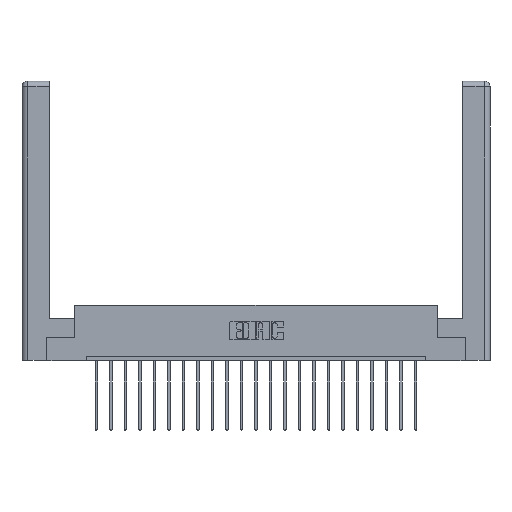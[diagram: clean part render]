
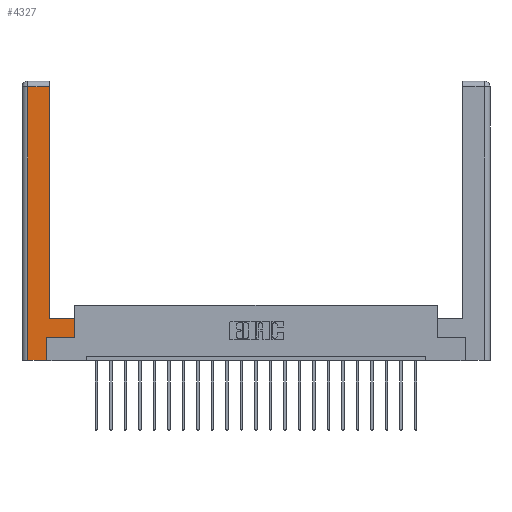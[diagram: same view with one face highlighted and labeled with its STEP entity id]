
A CAD part, top view. The second image highlights one B-rep face of the part: STEP entity #4327.
In plain terms, the highlighted planar face has unit normal (0, 0, 1).
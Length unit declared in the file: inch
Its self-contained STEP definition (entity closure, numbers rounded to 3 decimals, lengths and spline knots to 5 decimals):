
#248 = DIRECTION ( 'NONE',  ( -1., 0., 0. ) ) ;
#527 = DIRECTION ( 'NONE',  ( 1., 0., 0. ) ) ;
#644 = VERTEX_POINT ( 'NONE', #12038 ) ;
#904 = VERTEX_POINT ( 'NONE', #6009 ) ;
#1405 = ORIENTED_EDGE ( 'NONE', *, *, #10864, .T. ) ;
#1435 = CARTESIAN_POINT ( 'NONE',  ( 0.0615, 2.94, 0. ) ) ;
#1590 = LINE ( 'NONE', #9304, #5102 ) ;
#2837 = CARTESIAN_POINT ( 'NONE',  ( 0.295, 2.94, 0. ) ) ;
#3053 = VERTEX_POINT ( 'NONE', #1435 ) ;
#3635 = CARTESIAN_POINT ( 'NONE',  ( 0.0615, 2.94, 0. ) ) ;
#4297 = EDGE_CURVE ( 'NONE', #904, #19450, #11976, .T. ) ;
#4327 = ADVANCED_FACE ( 'NONE', ( #9293 ), #10858, .F. ) ;
#4337 = LINE ( 'NONE', #19168, #19892 ) ;
#4500 = ORIENTED_EDGE ( 'NONE', *, *, #20361, .T. ) ;
#5102 = VECTOR ( 'NONE', #7578, 39.37008 ) ;
#5104 = EDGE_CURVE ( 'NONE', #19450, #9506, #18352, .T. ) ;
#6009 = CARTESIAN_POINT ( 'NONE',  ( 0.265, 0., 0. ) ) ;
#6923 = CARTESIAN_POINT ( 'NONE',  ( 0.565, 0.45, 0. ) ) ;
#7255 = EDGE_LOOP ( 'NONE', ( #4500, #8034, #8121, #1405, #9281, #13465, #7885, #20680 ) ) ;
#7578 = DIRECTION ( 'NONE',  ( 0., 1., 0. ) ) ;
#7885 = ORIENTED_EDGE ( 'NONE', *, *, #19991, .T. ) ;
#8034 = ORIENTED_EDGE ( 'NONE', *, *, #12498, .T. ) ;
#8121 = ORIENTED_EDGE ( 'NONE', *, *, #20204, .T. ) ;
#8457 = CARTESIAN_POINT ( 'NONE',  ( 0.295, 0.45, 0. ) ) ;
#8510 = LINE ( 'NONE', #19008, #14132 ) ;
#8759 = VECTOR ( 'NONE', #17032, 39.37008 ) ;
#9281 = ORIENTED_EDGE ( 'NONE', *, *, #4297, .T. ) ;
#9293 = FACE_OUTER_BOUND ( 'NONE', #7255, .T. ) ;
#9304 = CARTESIAN_POINT ( 'NONE',  ( 0.295, 3., 0. ) ) ;
#9506 = VERTEX_POINT ( 'NONE', #20443 ) ;
#10354 = CARTESIAN_POINT ( 'NONE',  ( 0.265, 0.245, 0. ) ) ;
#10858 = PLANE ( 'NONE',  #19132 ) ;
#10864 = EDGE_CURVE ( 'NONE', #21640, #904, #8510, .T. ) ;
#11511 = LINE ( 'NONE', #3635, #16872 ) ;
#11976 = LINE ( 'NONE', #15924, #8759 ) ;
#12038 = CARTESIAN_POINT ( 'NONE',  ( 0.295, 0.45, 0. ) ) ;
#12167 = DIRECTION ( 'NONE',  ( 0., -1., 0. ) ) ;
#12498 = EDGE_CURVE ( 'NONE', #19823, #3053, #11511, .T. ) ;
#12790 = DIRECTION ( 'NONE',  ( -1., 0., 0. ) ) ;
#13465 = ORIENTED_EDGE ( 'NONE', *, *, #5104, .T. ) ;
#14132 = VECTOR ( 'NONE', #15485, 39.37008 ) ;
#14360 = VECTOR ( 'NONE', #15308, 39.37008 ) ;
#15308 = DIRECTION ( 'NONE',  ( -1., 0., 0. ) ) ;
#15485 = DIRECTION ( 'NONE',  ( 1., 0., 0. ) ) ;
#15876 = VECTOR ( 'NONE', #16725, 39.37008 ) ;
#15924 = CARTESIAN_POINT ( 'NONE',  ( 0.265, 0.245, 0. ) ) ;
#16725 = DIRECTION ( 'NONE',  ( 0., 1., 0. ) ) ;
#16872 = VECTOR ( 'NONE', #248, 39.37008 ) ;
#16963 = CARTESIAN_POINT ( 'NONE',  ( 0.0615, 0., 0. ) ) ;
#17032 = DIRECTION ( 'NONE',  ( 0., 1., 0. ) ) ;
#17434 = CARTESIAN_POINT ( 'NONE',  ( 0., 0., 0. ) ) ;
#18323 = EDGE_CURVE ( 'NONE', #20527, #644, #20216, .T. ) ;
#18352 = LINE ( 'NONE', #21025, #21838 ) ;
#19008 = CARTESIAN_POINT ( 'NONE',  ( 0.265, 0., 0. ) ) ;
#19132 = AXIS2_PLACEMENT_3D ( 'NONE', #17434, #19445, #12790 ) ;
#19168 = CARTESIAN_POINT ( 'NONE',  ( 0.0615, 0., 0. ) ) ;
#19445 = DIRECTION ( 'NONE',  ( 0., 0., -1. ) ) ;
#19450 = VERTEX_POINT ( 'NONE', #10354 ) ;
#19823 = VERTEX_POINT ( 'NONE', #2837 ) ;
#19892 = VECTOR ( 'NONE', #12167, 39.37008 ) ;
#19991 = EDGE_CURVE ( 'NONE', #9506, #20527, #20428, .T. ) ;
#20204 = EDGE_CURVE ( 'NONE', #3053, #21640, #4337, .T. ) ;
#20216 = LINE ( 'NONE', #8457, #14360 ) ;
#20315 = CARTESIAN_POINT ( 'NONE',  ( 0.565, 0.45, 0. ) ) ;
#20361 = EDGE_CURVE ( 'NONE', #644, #19823, #1590, .T. ) ;
#20428 = LINE ( 'NONE', #20315, #15876 ) ;
#20443 = CARTESIAN_POINT ( 'NONE',  ( 0.565, 0.245, 0. ) ) ;
#20527 = VERTEX_POINT ( 'NONE', #6923 ) ;
#20680 = ORIENTED_EDGE ( 'NONE', *, *, #18323, .T. ) ;
#21025 = CARTESIAN_POINT ( 'NONE',  ( 0.565, 0.245, 0. ) ) ;
#21640 = VERTEX_POINT ( 'NONE', #16963 ) ;
#21838 = VECTOR ( 'NONE', #527, 39.37008 ) ;
